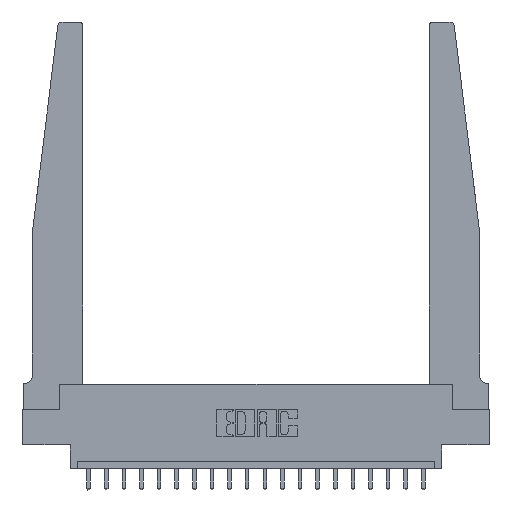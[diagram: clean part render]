
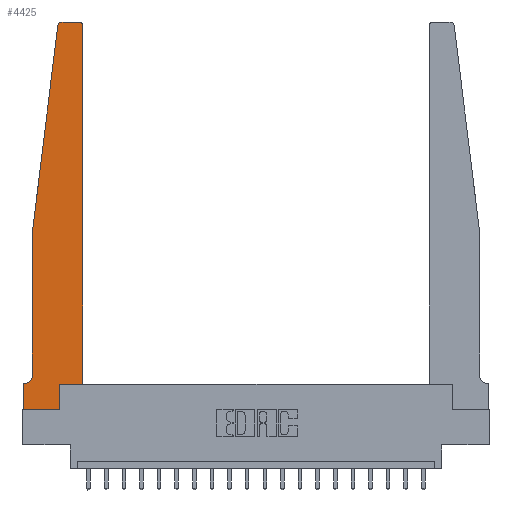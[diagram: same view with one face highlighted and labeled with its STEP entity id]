
A CAD part, top view. The second image highlights one B-rep face of the part: STEP entity #4425.
In plain terms, the highlighted planar face has unit normal (0, 0, 1).
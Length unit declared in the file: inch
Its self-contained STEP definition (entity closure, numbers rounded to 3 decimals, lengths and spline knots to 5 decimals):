
#713 = EDGE_CURVE ( 'NONE', #16351, #13123, #13269, .T. ) ;
#891 = VERTEX_POINT ( 'NONE', #17257 ) ;
#1149 = ORIENTED_EDGE ( 'NONE', *, *, #11576, .T. ) ;
#1342 = VERTEX_POINT ( 'NONE', #3989 ) ;
#1383 = VECTOR ( 'NONE', #16979, 39.37008 ) ;
#1519 = DIRECTION ( 'NONE',  ( 0., -1., 0. ) ) ;
#1635 = CARTESIAN_POINT ( 'NONE',  ( 0.015, 0.2375, 0.37 ) ) ;
#1695 = CARTESIAN_POINT ( 'NONE',  ( 0.2605, 0., 0.37 ) ) ;
#2122 = LINE ( 'NONE', #6164, #1383 ) ;
#2147 = CIRCLE ( 'NONE', #12401, 0.03 ) ;
#2180 = FACE_OUTER_BOUND ( 'NONE', #8543, .T. ) ;
#2267 = VECTOR ( 'NONE', #1519, 39.37008 ) ;
#2827 = CARTESIAN_POINT ( 'NONE',  ( 0.25, 2.75, 0.37 ) ) ;
#2887 = VERTEX_POINT ( 'NONE', #4794 ) ;
#2908 = VERTEX_POINT ( 'NONE', #16893 ) ;
#2972 = ORIENTED_EDGE ( 'NONE', *, *, #16176, .T. ) ;
#3046 = CARTESIAN_POINT ( 'NONE',  ( 0., 0., 0.37 ) ) ;
#3171 = LINE ( 'NONE', #14147, #18846 ) ;
#3179 = DIRECTION ( 'NONE',  ( 0., 1., 0. ) ) ;
#3219 = DIRECTION ( 'NONE',  ( 0., 0., -1. ) ) ;
#3529 = PLANE ( 'NONE',  #4757 ) ;
#3877 = DIRECTION ( 'NONE',  ( 1., 0., 0. ) ) ;
#3989 = CARTESIAN_POINT ( 'NONE',  ( 0.425, 0.18, 0.37 ) ) ;
#4292 = VECTOR ( 'NONE', #12403, 39.37008 ) ;
#4407 = DIRECTION ( 'NONE',  ( 0., -1., 0. ) ) ;
#4425 = ADVANCED_FACE ( 'NONE', ( #2180 ), #3529, .T. ) ;
#4719 = AXIS2_PLACEMENT_3D ( 'NONE', #1635, #3219, #18570 ) ;
#4757 = AXIS2_PLACEMENT_3D ( 'NONE', #12880, #14530, #19188 ) ;
#4794 = CARTESIAN_POINT ( 'NONE',  ( 0.2605, 0.18, 0.37 ) ) ;
#5066 = AXIS2_PLACEMENT_3D ( 'NONE', #5428, #10056, #5488 ) ;
#5372 = VERTEX_POINT ( 'NONE', #19298 ) ;
#5428 = CARTESIAN_POINT ( 'NONE',  ( 0.27653, 2.72, 0.37 ) ) ;
#5463 = LINE ( 'NONE', #3046, #2267 ) ;
#5488 = DIRECTION ( 'NONE',  ( 1., 0., 0. ) ) ;
#5616 = CIRCLE ( 'NONE', #4719, 0.05 ) ;
#6159 = ORIENTED_EDGE ( 'NONE', *, *, #19233, .T. ) ;
#6164 = CARTESIAN_POINT ( 'NONE',  ( 0.425, 0.18, 0.37 ) ) ;
#6933 = EDGE_CURVE ( 'NONE', #10682, #891, #18469, .T. ) ;
#6969 = ORIENTED_EDGE ( 'NONE', *, *, #713, .T. ) ;
#7013 = CARTESIAN_POINT ( 'NONE',  ( 0.065, 1.25, 0.37 ) ) ;
#7788 = VECTOR ( 'NONE', #19874, 39.37008 ) ;
#8103 = ORIENTED_EDGE ( 'NONE', *, *, #12928, .T. ) ;
#8486 = VECTOR ( 'NONE', #17061, 39.37008 ) ;
#8543 = EDGE_LOOP ( 'NONE', ( #6159, #14539, #15681, #1149, #9289, #9430, #2972, #6969, #18738, #17593, #8103, #17373 ) ) ;
#8650 = LINE ( 'NONE', #9527, #12290 ) ;
#9099 = VECTOR ( 'NONE', #16991, 39.37008 ) ;
#9289 = ORIENTED_EDGE ( 'NONE', *, *, #18471, .T. ) ;
#9430 = ORIENTED_EDGE ( 'NONE', *, *, #6933, .T. ) ;
#9527 = CARTESIAN_POINT ( 'NONE',  ( 0.065, 1.25, 0.37 ) ) ;
#9676 = VERTEX_POINT ( 'NONE', #19718 ) ;
#9814 = CARTESIAN_POINT ( 'NONE',  ( 0.24675, 2.72367, 0.37 ) ) ;
#9999 = CARTESIAN_POINT ( 'NONE',  ( 0.015, 0.1875, 0.37 ) ) ;
#10056 = DIRECTION ( 'NONE',  ( 0., 0., 1. ) ) ;
#10454 = VECTOR ( 'NONE', #3179, 39.37008 ) ;
#10682 = VERTEX_POINT ( 'NONE', #9999 ) ;
#10704 = CARTESIAN_POINT ( 'NONE',  ( 0.065, 0.1875, 0.37 ) ) ;
#10785 = CIRCLE ( 'NONE', #5066, 0.03 ) ;
#11576 = EDGE_CURVE ( 'NONE', #18938, #9676, #3171, .T. ) ;
#11997 = CARTESIAN_POINT ( 'NONE',  ( 0.395, 2.75, 0.37 ) ) ;
#12290 = VECTOR ( 'NONE', #16188, 39.37008 ) ;
#12401 = AXIS2_PLACEMENT_3D ( 'NONE', #16506, #19598, #3877 ) ;
#12403 = DIRECTION ( 'NONE',  ( -1., 0., 0. ) ) ;
#12488 = VERTEX_POINT ( 'NONE', #11997 ) ;
#12880 = CARTESIAN_POINT ( 'NONE',  ( 0., 0.1875, 0.37 ) ) ;
#12928 = EDGE_CURVE ( 'NONE', #1342, #2908, #14856, .T. ) ;
#13018 = EDGE_CURVE ( 'NONE', #2887, #1342, #2122, .T. ) ;
#13123 = VERTEX_POINT ( 'NONE', #1695 ) ;
#13235 = CARTESIAN_POINT ( 'NONE',  ( 0., 0., 0.37 ) ) ;
#13269 = LINE ( 'NONE', #20057, #9099 ) ;
#13559 = VERTEX_POINT ( 'NONE', #9814 ) ;
#14147 = CARTESIAN_POINT ( 'NONE',  ( 0.065, 1.25, 0.37 ) ) ;
#14384 = LINE ( 'NONE', #20001, #7788 ) ;
#14530 = DIRECTION ( 'NONE',  ( 0., 0., 1. ) ) ;
#14539 = ORIENTED_EDGE ( 'NONE', *, *, #17068, .T. ) ;
#14856 = LINE ( 'NONE', #15810, #10454 ) ;
#15681 = ORIENTED_EDGE ( 'NONE', *, *, #16017, .T. ) ;
#15810 = CARTESIAN_POINT ( 'NONE',  ( 0.425, 0.18, 0.37 ) ) ;
#16017 = EDGE_CURVE ( 'NONE', #13559, #18938, #8650, .T. ) ;
#16176 = EDGE_CURVE ( 'NONE', #891, #16351, #5463, .T. ) ;
#16188 = DIRECTION ( 'NONE',  ( -0.122, -0.992, 0. ) ) ;
#16316 = LINE ( 'NONE', #2827, #8486 ) ;
#16351 = VERTEX_POINT ( 'NONE', #13235 ) ;
#16506 = CARTESIAN_POINT ( 'NONE',  ( 0.395, 2.72, 0.37 ) ) ;
#16893 = CARTESIAN_POINT ( 'NONE',  ( 0.425, 2.72, 0.37 ) ) ;
#16979 = DIRECTION ( 'NONE',  ( 1., 0., 0. ) ) ;
#16991 = DIRECTION ( 'NONE',  ( 1., 0., 0. ) ) ;
#17061 = DIRECTION ( 'NONE',  ( -1., 0., 0. ) ) ;
#17068 = EDGE_CURVE ( 'NONE', #5372, #13559, #10785, .T. ) ;
#17257 = CARTESIAN_POINT ( 'NONE',  ( 0., 0.1875, 0.37 ) ) ;
#17373 = ORIENTED_EDGE ( 'NONE', *, *, #19030, .T. ) ;
#17593 = ORIENTED_EDGE ( 'NONE', *, *, #13018, .T. ) ;
#18469 = LINE ( 'NONE', #10704, #4292 ) ;
#18471 = EDGE_CURVE ( 'NONE', #9676, #10682, #5616, .T. ) ;
#18570 = DIRECTION ( 'NONE',  ( -1., 0., 0. ) ) ;
#18738 = ORIENTED_EDGE ( 'NONE', *, *, #18839, .T. ) ;
#18839 = EDGE_CURVE ( 'NONE', #13123, #2887, #14384, .T. ) ;
#18846 = VECTOR ( 'NONE', #4407, 39.37008 ) ;
#18938 = VERTEX_POINT ( 'NONE', #7013 ) ;
#19030 = EDGE_CURVE ( 'NONE', #2908, #12488, #2147, .T. ) ;
#19188 = DIRECTION ( 'NONE',  ( 1., 0., 0. ) ) ;
#19233 = EDGE_CURVE ( 'NONE', #12488, #5372, #16316, .T. ) ;
#19298 = CARTESIAN_POINT ( 'NONE',  ( 0.27653, 2.75, 0.37 ) ) ;
#19598 = DIRECTION ( 'NONE',  ( 0., 0., 1. ) ) ;
#19718 = CARTESIAN_POINT ( 'NONE',  ( 0.065, 0.2375, 0.37 ) ) ;
#19874 = DIRECTION ( 'NONE',  ( 0., 1., 0. ) ) ;
#20001 = CARTESIAN_POINT ( 'NONE',  ( 0.2605, 0.18, 0.37 ) ) ;
#20057 = CARTESIAN_POINT ( 'NONE',  ( 0., 0., 0.37 ) ) ;
